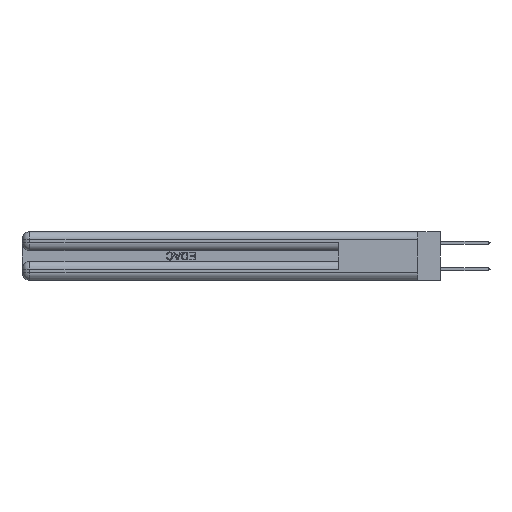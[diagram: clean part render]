
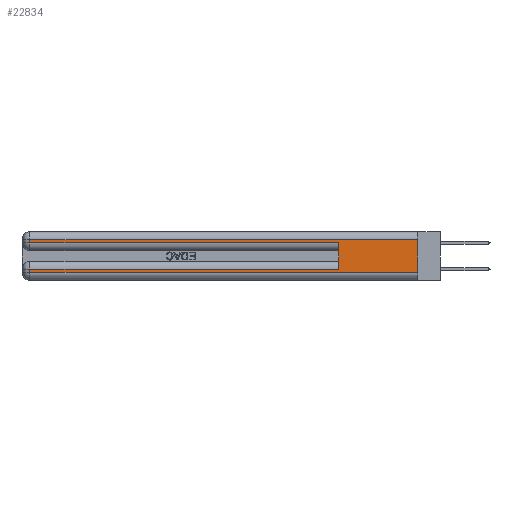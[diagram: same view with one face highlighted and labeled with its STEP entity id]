
A CAD part, left-side view. The second image highlights one B-rep face of the part: STEP entity #22834.
In plain terms, the highlighted planar face has unit normal (-1, 0, 0).
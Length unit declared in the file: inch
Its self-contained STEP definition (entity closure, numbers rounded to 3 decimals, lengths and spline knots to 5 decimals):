
#531 = VERTEX_POINT ( 'NONE', #24181 ) ;
#3786 = VERTEX_POINT ( 'NONE', #25639 ) ;
#5002 = LINE ( 'NONE', #26973, #42834 ) ;
#5172 = LINE ( 'NONE', #6844, #23694 ) ;
#5409 = ORIENTED_EDGE ( 'NONE', *, *, #18302, .T. ) ;
#5740 = VECTOR ( 'NONE', #15366, 39.37008 ) ;
#5773 = VERTEX_POINT ( 'NONE', #21893 ) ;
#6404 = VERTEX_POINT ( 'NONE', #10372 ) ;
#6844 = CARTESIAN_POINT ( 'NONE',  ( 0., 0., 0.37 ) ) ;
#7151 = EDGE_CURVE ( 'NONE', #5773, #12452, #16785, .T. ) ;
#7512 = DIRECTION ( 'NONE',  ( 0., 0., -1. ) ) ;
#8822 = CARTESIAN_POINT ( 'NONE',  ( 0., 0., 0.06 ) ) ;
#9850 = DIRECTION ( 'NONE',  ( 0., 0., -1. ) ) ;
#10372 = CARTESIAN_POINT ( 'NONE',  ( 0., 0., 0.31 ) ) ;
#12452 = VERTEX_POINT ( 'NONE', #19938 ) ;
#13461 = EDGE_CURVE ( 'NONE', #14665, #3786, #27412, .T. ) ;
#13490 = CARTESIAN_POINT ( 'NONE',  ( 0., 0., 0.37 ) ) ;
#13764 = VECTOR ( 'NONE', #18514, 39.37008 ) ;
#14637 = VECTOR ( 'NONE', #9850, 39.37008 ) ;
#14665 = VERTEX_POINT ( 'NONE', #17224 ) ;
#15273 = VECTOR ( 'NONE', #32043, 39.37008 ) ;
#15366 = DIRECTION ( 'NONE',  ( 0., 0., 1. ) ) ;
#16160 = EDGE_CURVE ( 'NONE', #6404, #26915, #5172, .T. ) ;
#16785 = LINE ( 'NONE', #22754, #5740 ) ;
#16967 = LINE ( 'NONE', #24555, #14637 ) ;
#17224 = CARTESIAN_POINT ( 'NONE',  ( 0., 2.94, 0.31 ) ) ;
#17234 = DIRECTION ( 'NONE',  ( 0., 0., -1. ) ) ;
#17279 = CARTESIAN_POINT ( 'NONE',  ( 0., 0., 0.085 ) ) ;
#17406 = FACE_OUTER_BOUND ( 'NONE', #36362, .T. ) ;
#17640 = VECTOR ( 'NONE', #7512, 39.37008 ) ;
#18302 = EDGE_CURVE ( 'NONE', #43184, #26915, #5002, .T. ) ;
#18328 = ORIENTED_EDGE ( 'NONE', *, *, #20207, .T. ) ;
#18514 = DIRECTION ( 'NONE',  ( 0., -1., 0. ) ) ;
#19938 = CARTESIAN_POINT ( 'NONE',  ( 0., 0.6, 0.285 ) ) ;
#20207 = EDGE_CURVE ( 'NONE', #6404, #14665, #39292, .T. ) ;
#20289 = EDGE_CURVE ( 'NONE', #5773, #531, #44334, .T. ) ;
#21893 = CARTESIAN_POINT ( 'NONE',  ( 0., 0.6, 0.085 ) ) ;
#22754 = CARTESIAN_POINT ( 'NONE',  ( 0., 0.6, 0.145 ) ) ;
#22834 = ADVANCED_FACE ( 'NONE', ( #17406 ), #35464, .F. ) ;
#23694 = VECTOR ( 'NONE', #28963, 39.37008 ) ;
#24181 = CARTESIAN_POINT ( 'NONE',  ( 0., 2.94, 0.085 ) ) ;
#24555 = CARTESIAN_POINT ( 'NONE',  ( 0., 2.94, 0.37 ) ) ;
#24971 = CARTESIAN_POINT ( 'NONE',  ( 0., 2.94, 0.06 ) ) ;
#25639 = CARTESIAN_POINT ( 'NONE',  ( 0., 2.94, 0.285 ) ) ;
#26915 = VERTEX_POINT ( 'NONE', #8822 ) ;
#26973 = CARTESIAN_POINT ( 'NONE',  ( 0., 0., 0.06 ) ) ;
#27412 = LINE ( 'NONE', #33124, #17640 ) ;
#28963 = DIRECTION ( 'NONE',  ( 0., 0., -1. ) ) ;
#29703 = ORIENTED_EDGE ( 'NONE', *, *, #20289, .T. ) ;
#29850 = ORIENTED_EDGE ( 'NONE', *, *, #13461, .T. ) ;
#30660 = ORIENTED_EDGE ( 'NONE', *, *, #36908, .T. ) ;
#30694 = DIRECTION ( 'NONE',  ( 0., -1., 0. ) ) ;
#31938 = ORIENTED_EDGE ( 'NONE', *, *, #33241, .T. ) ;
#32043 = DIRECTION ( 'NONE',  ( 0., 1., 0. ) ) ;
#32265 = ORIENTED_EDGE ( 'NONE', *, *, #7151, .F. ) ;
#33124 = CARTESIAN_POINT ( 'NONE',  ( 0., 2.94, 0.37 ) ) ;
#33241 = EDGE_CURVE ( 'NONE', #531, #43184, #16967, .T. ) ;
#35464 = PLANE ( 'NONE',  #45087 ) ;
#36362 = EDGE_LOOP ( 'NONE', ( #44356, #18328, #29850, #30660, #32265, #29703, #31938, #5409 ) ) ;
#36908 = EDGE_CURVE ( 'NONE', #3786, #12452, #44021, .T. ) ;
#38134 = VECTOR ( 'NONE', #45886, 39.37008 ) ;
#39094 = DIRECTION ( 'NONE',  ( 1., 0., 0. ) ) ;
#39292 = LINE ( 'NONE', #42292, #38134 ) ;
#42292 = CARTESIAN_POINT ( 'NONE',  ( 0., 0., 0.31 ) ) ;
#42834 = VECTOR ( 'NONE', #30694, 39.37008 ) ;
#43184 = VERTEX_POINT ( 'NONE', #24971 ) ;
#43801 = CARTESIAN_POINT ( 'NONE',  ( 0., 0., 0.285 ) ) ;
#44021 = LINE ( 'NONE', #43801, #13764 ) ;
#44334 = LINE ( 'NONE', #17279, #15273 ) ;
#44356 = ORIENTED_EDGE ( 'NONE', *, *, #16160, .F. ) ;
#45087 = AXIS2_PLACEMENT_3D ( 'NONE', #13490, #39094, #17234 ) ;
#45886 = DIRECTION ( 'NONE',  ( 0., 1., 0. ) ) ;
